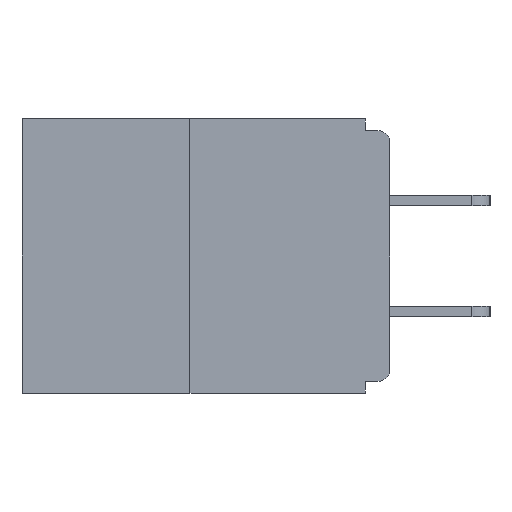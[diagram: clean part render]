
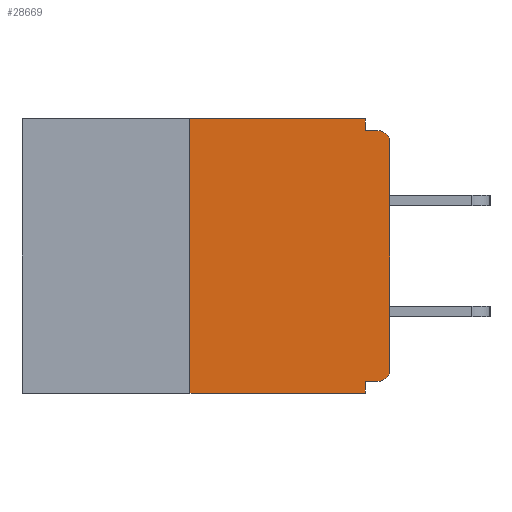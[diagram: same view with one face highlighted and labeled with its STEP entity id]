
A CAD part, left-side view. The second image highlights one B-rep face of the part: STEP entity #28669.
In plain terms, the highlighted planar face has unit normal (-1, 0, 0).
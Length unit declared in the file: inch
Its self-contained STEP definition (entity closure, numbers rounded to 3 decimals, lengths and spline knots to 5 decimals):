
#147 = VECTOR ( 'NONE', #2020, 39.37008 ) ;
#339 = EDGE_CURVE ( 'NONE', #20616, #23626, #11200, .T. ) ;
#450 = VECTOR ( 'NONE', #6211, 39.37008 ) ;
#1145 = CARTESIAN_POINT ( 'NONE',  ( 0., 0.25, 0. ) ) ;
#1794 = CARTESIAN_POINT ( 'NONE',  ( 0., 0.015, -0.03 ) ) ;
#2010 = CARTESIAN_POINT ( 'NONE',  ( 0., 0., -0.015 ) ) ;
#2020 = DIRECTION ( 'NONE',  ( 0., 1., 0. ) ) ;
#2151 = DIRECTION ( 'NONE',  ( 0., -1., 0. ) ) ;
#2196 = CARTESIAN_POINT ( 'NONE',  ( 0., 0.031, -0.015 ) ) ;
#2457 = EDGE_CURVE ( 'NONE', #12689, #28101, #8459, .T. ) ;
#2533 = VERTEX_POINT ( 'NONE', #18624 ) ;
#3457 = CARTESIAN_POINT ( 'NONE',  ( 0., 0.25, 0. ) ) ;
#3574 = LINE ( 'NONE', #13239, #19668 ) ;
#3809 = CARTESIAN_POINT ( 'NONE',  ( 0., 0.46, -0.343 ) ) ;
#4016 = DIRECTION ( 'NONE',  ( 0., 0., -1. ) ) ;
#5020 = CARTESIAN_POINT ( 'NONE',  ( 0., 0., 0. ) ) ;
#5527 = CARTESIAN_POINT ( 'NONE',  ( 0., 0.46, 0. ) ) ;
#5612 = CARTESIAN_POINT ( 'NONE',  ( 0., 0.031, -0.328 ) ) ;
#6211 = DIRECTION ( 'NONE',  ( 0., 0., 1. ) ) ;
#6280 = VERTEX_POINT ( 'NONE', #23778 ) ;
#6361 = EDGE_CURVE ( 'NONE', #28395, #2533, #8060, .T. ) ;
#6755 = LINE ( 'NONE', #2010, #10477 ) ;
#7228 = DIRECTION ( 'NONE',  ( 0., 0., 1. ) ) ;
#7788 = EDGE_CURVE ( 'NONE', #17283, #6280, #25547, .T. ) ;
#7924 = DIRECTION ( 'NONE',  ( 0., 0., -1. ) ) ;
#8060 = LINE ( 'NONE', #5527, #13423 ) ;
#8459 = CIRCLE ( 'NONE', #31287, 0.015 ) ;
#8878 = DIRECTION ( 'NONE',  ( 1., 0., 0. ) ) ;
#9611 = LINE ( 'NONE', #5020, #10304 ) ;
#9888 = CARTESIAN_POINT ( 'NONE',  ( 0., 0., -0.03 ) ) ;
#10304 = VECTOR ( 'NONE', #7228, 39.37008 ) ;
#10327 = CARTESIAN_POINT ( 'NONE',  ( 0., 0.015, -0.328 ) ) ;
#10477 = VECTOR ( 'NONE', #2151, 39.37008 ) ;
#11051 = EDGE_CURVE ( 'NONE', #2533, #20090, #21705, .T. ) ;
#11200 = LINE ( 'NONE', #18679, #147 ) ;
#11782 = ORIENTED_EDGE ( 'NONE', *, *, #6361, .F. ) ;
#12663 = EDGE_CURVE ( 'NONE', #20090, #28101, #6755, .T. ) ;
#12689 = VERTEX_POINT ( 'NONE', #9888 ) ;
#12913 = DIRECTION ( 'NONE',  ( 0., 0., -1. ) ) ;
#13239 = CARTESIAN_POINT ( 'NONE',  ( 0., 0.031, -0.343 ) ) ;
#13423 = VECTOR ( 'NONE', #29640, 39.37008 ) ;
#13482 = DIRECTION ( 'NONE',  ( 0., -1., 0. ) ) ;
#13553 = DIRECTION ( 'NONE',  ( -1., 0., 0. ) ) ;
#14272 = EDGE_CURVE ( 'NONE', #17283, #28395, #17957, .T. ) ;
#15086 = EDGE_CURVE ( 'NONE', #23626, #6280, #3574, .T. ) ;
#15884 = CARTESIAN_POINT ( 'NONE',  ( 0., 0.25, -0.343 ) ) ;
#16339 = CARTESIAN_POINT ( 'NONE',  ( 0., 0., -0.313 ) ) ;
#16930 = CARTESIAN_POINT ( 'NONE',  ( 0., 0.015, -0.015 ) ) ;
#17283 = VERTEX_POINT ( 'NONE', #15884 ) ;
#17568 = AXIS2_PLACEMENT_3D ( 'NONE', #27679, #8878, #12913 ) ;
#17957 = LINE ( 'NONE', #1145, #450 ) ;
#18624 = CARTESIAN_POINT ( 'NONE',  ( 0., 0.031, 0. ) ) ;
#18679 = CARTESIAN_POINT ( 'NONE',  ( 0., 0., -0.328 ) ) ;
#19371 = AXIS2_PLACEMENT_3D ( 'NONE', #30009, #26827, #7924 ) ;
#19583 = FACE_OUTER_BOUND ( 'NONE', #20388, .T. ) ;
#19668 = VECTOR ( 'NONE', #25449, 39.37008 ) ;
#20090 = VERTEX_POINT ( 'NONE', #2196 ) ;
#20388 = EDGE_LOOP ( 'NONE', ( #11782, #28939, #28858, #26535, #22980, #26309, #25400, #22809, #28863, #29044 ) ) ;
#20616 = VERTEX_POINT ( 'NONE', #10327 ) ;
#21705 = LINE ( 'NONE', #29011, #26146 ) ;
#22626 = VECTOR ( 'NONE', #13482, 39.37008 ) ;
#22809 = ORIENTED_EDGE ( 'NONE', *, *, #2457, .T. ) ;
#22980 = ORIENTED_EDGE ( 'NONE', *, *, #339, .F. ) ;
#23232 = DIRECTION ( 'NONE',  ( 0., 0., -1. ) ) ;
#23626 = VERTEX_POINT ( 'NONE', #5612 ) ;
#23778 = CARTESIAN_POINT ( 'NONE',  ( 0., 0.031, -0.343 ) ) ;
#24323 = EDGE_CURVE ( 'NONE', #27903, #12689, #9611, .T. ) ;
#25400 = ORIENTED_EDGE ( 'NONE', *, *, #24323, .T. ) ;
#25449 = DIRECTION ( 'NONE',  ( 0., 0., -1. ) ) ;
#25547 = LINE ( 'NONE', #3809, #22626 ) ;
#26146 = VECTOR ( 'NONE', #4016, 39.37008 ) ;
#26309 = ORIENTED_EDGE ( 'NONE', *, *, #29050, .T. ) ;
#26535 = ORIENTED_EDGE ( 'NONE', *, *, #15086, .F. ) ;
#26827 = DIRECTION ( 'NONE',  ( -1., 0., 0. ) ) ;
#26993 = CIRCLE ( 'NONE', #19371, 0.015 ) ;
#27679 = CARTESIAN_POINT ( 'NONE',  ( 0., 0.46, 0. ) ) ;
#27903 = VERTEX_POINT ( 'NONE', #16339 ) ;
#28101 = VERTEX_POINT ( 'NONE', #16930 ) ;
#28395 = VERTEX_POINT ( 'NONE', #3457 ) ;
#28669 = ADVANCED_FACE ( 'NONE', ( #19583 ), #29288, .F. ) ;
#28858 = ORIENTED_EDGE ( 'NONE', *, *, #7788, .T. ) ;
#28863 = ORIENTED_EDGE ( 'NONE', *, *, #12663, .F. ) ;
#28939 = ORIENTED_EDGE ( 'NONE', *, *, #14272, .F. ) ;
#29011 = CARTESIAN_POINT ( 'NONE',  ( 0., 0.031, 0. ) ) ;
#29044 = ORIENTED_EDGE ( 'NONE', *, *, #11051, .F. ) ;
#29050 = EDGE_CURVE ( 'NONE', #20616, #27903, #26993, .T. ) ;
#29288 = PLANE ( 'NONE',  #17568 ) ;
#29640 = DIRECTION ( 'NONE',  ( 0., -1., 0. ) ) ;
#30009 = CARTESIAN_POINT ( 'NONE',  ( 0., 0.015, -0.313 ) ) ;
#31287 = AXIS2_PLACEMENT_3D ( 'NONE', #1794, #13553, #23232 ) ;
